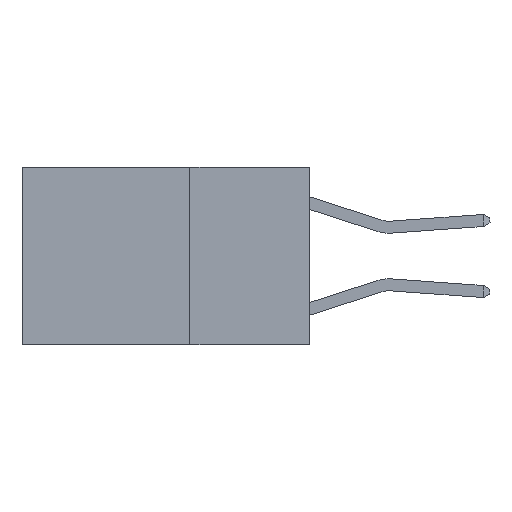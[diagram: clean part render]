
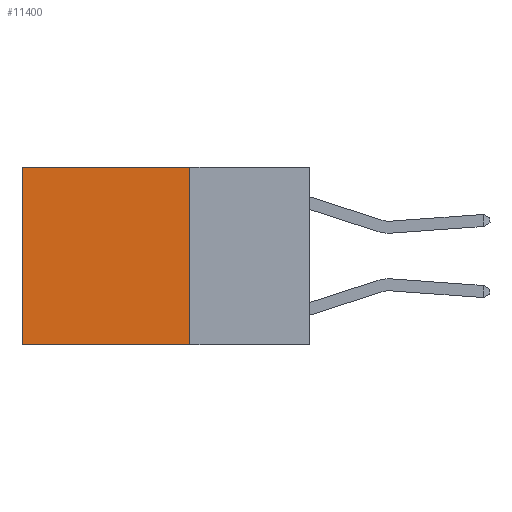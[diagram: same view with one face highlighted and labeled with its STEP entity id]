
A CAD part, left-side view. The second image highlights one B-rep face of the part: STEP entity #11400.
In plain terms, the highlighted planar face has unit normal (-1, 0, 0).
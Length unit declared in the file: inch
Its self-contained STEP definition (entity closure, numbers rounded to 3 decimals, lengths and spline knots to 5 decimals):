
#78 = CARTESIAN_POINT ( 'NONE',  ( 0.2625, 0.25, 0. ) ) ;
#123 = CARTESIAN_POINT ( 'NONE',  ( 0.2625, 0.6, 0. ) ) ;
#405 = DIRECTION ( 'NONE',  ( 0., 1., 0. ) ) ;
#1308 = DIRECTION ( 'NONE',  ( 0., 0., -1. ) ) ;
#1465 = EDGE_CURVE ( 'NONE', #3966, #7648, #6269, .T. ) ;
#1519 = ORIENTED_EDGE ( 'NONE', *, *, #6788, .F. ) ;
#1585 = LINE ( 'NONE', #14204, #15460 ) ;
#2915 = CARTESIAN_POINT ( 'NONE',  ( 0.2625, 0.25, 0. ) ) ;
#3695 = VECTOR ( 'NONE', #15352, 39.37008 ) ;
#3750 = PLANE ( 'NONE',  #10250 ) ;
#3966 = VERTEX_POINT ( 'NONE', #2915 ) ;
#5421 = VERTEX_POINT ( 'NONE', #13423 ) ;
#6258 = VERTEX_POINT ( 'NONE', #16055 ) ;
#6269 = LINE ( 'NONE', #14329, #3695 ) ;
#6638 = ORIENTED_EDGE ( 'NONE', *, *, #13067, .F. ) ;
#6666 = VECTOR ( 'NONE', #10261, 39.37008 ) ;
#6788 = EDGE_CURVE ( 'NONE', #6258, #5421, #1585, .T. ) ;
#7024 = LINE ( 'NONE', #123, #9560 ) ;
#7046 = CARTESIAN_POINT ( 'NONE',  ( 0.2625, 0.6, 0. ) ) ;
#7563 = DIRECTION ( 'NONE',  ( 1., 0., 0. ) ) ;
#7648 = VERTEX_POINT ( 'NONE', #7046 ) ;
#8018 = ORIENTED_EDGE ( 'NONE', *, *, #15791, .T. ) ;
#9560 = VECTOR ( 'NONE', #12440, 39.37008 ) ;
#10003 = LINE ( 'NONE', #78, #6666 ) ;
#10250 = AXIS2_PLACEMENT_3D ( 'NONE', #14956, #7563, #1308 ) ;
#10261 = DIRECTION ( 'NONE',  ( 0., 0., -1. ) ) ;
#11400 = ADVANCED_FACE ( 'NONE', ( #11761 ), #3750, .F. ) ;
#11761 = FACE_OUTER_BOUND ( 'NONE', #13849, .T. ) ;
#12440 = DIRECTION ( 'NONE',  ( 0., 0., -1. ) ) ;
#13067 = EDGE_CURVE ( 'NONE', #3966, #6258, #10003, .T. ) ;
#13423 = CARTESIAN_POINT ( 'NONE',  ( 0.2625, 0.6, -0.37 ) ) ;
#13849 = EDGE_LOOP ( 'NONE', ( #8018, #1519, #6638, #13965 ) ) ;
#13965 = ORIENTED_EDGE ( 'NONE', *, *, #1465, .T. ) ;
#14204 = CARTESIAN_POINT ( 'NONE',  ( 0.2625, 0.25, -0.37 ) ) ;
#14329 = CARTESIAN_POINT ( 'NONE',  ( 0.2625, 0.25, 0. ) ) ;
#14956 = CARTESIAN_POINT ( 'NONE',  ( 0.2625, 0.25, 0. ) ) ;
#15352 = DIRECTION ( 'NONE',  ( 0., 1., 0. ) ) ;
#15460 = VECTOR ( 'NONE', #405, 39.37008 ) ;
#15791 = EDGE_CURVE ( 'NONE', #7648, #5421, #7024, .T. ) ;
#16055 = CARTESIAN_POINT ( 'NONE',  ( 0.2625, 0.25, -0.37 ) ) ;
